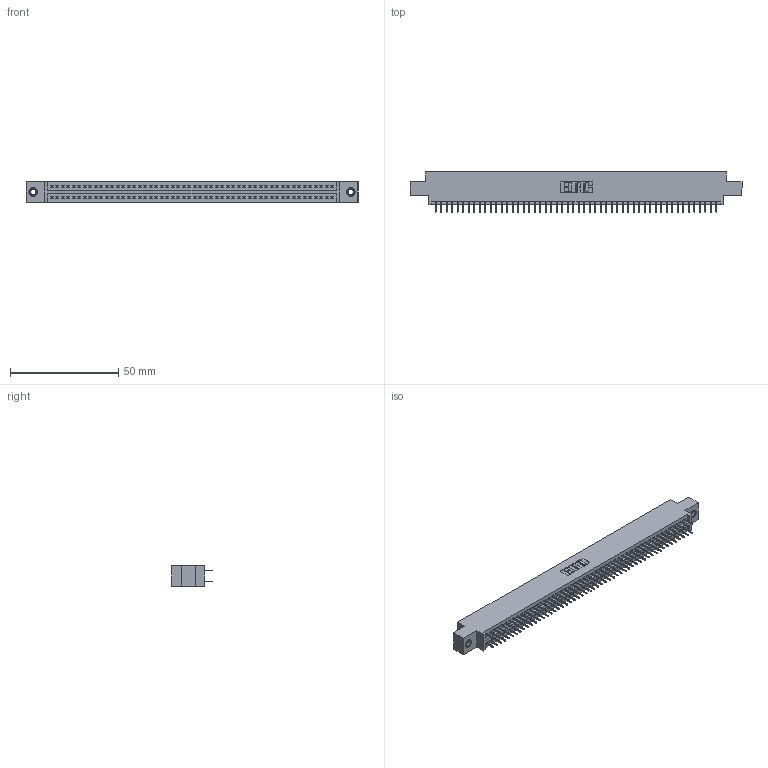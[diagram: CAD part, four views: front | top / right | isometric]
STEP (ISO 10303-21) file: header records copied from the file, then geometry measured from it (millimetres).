
FILE_DESCRIPTION (( 'STEP AP203' ), '1' );
FILE_NAME ('345-104-525-807.STEP', '2020-09-21T19:34:53', ( '' ), ( '' ), 'SwSTEP 2.0', 'SolidWorks 2020', '' );
FILE_SCHEMA (( 'CONFIG_CONTROL_DESIGN' ));
Length unit declared in the file: inch
Products named in the file (4): 345 Part_0.170 Offset - 0.156 Dia-TI; 345-250-001_345-250-005-103; 345-104-525-807; 345-292-001_345-293-125
Assembly tree (107 placements, depth 2):
  345-104-525-807
    345 Part_0.170 Offset - 0.156 Dia-TI
    345-292-001_345-293-125  x104
    345-250-001_345-250-005-103  x2
Bounding box: 153.29 x 18.72 x 9.4 mm (x, y, z)
Volume: 14685.4 mm3; surface area: 21556.7 mm2
Topology: 107 solids, 107 shells, 5806 faces, 16401 edges, 10510 vertices
Faces by surface type: plane 4172, cylinder 1618, cone 12, torus 4
Entity records: 40846 total; most frequent: CARTESIAN_POINT 6819, ORIENTED_EDGE 6746, DIRECTION 6027, EDGE_CURVE 3373, VECTOR 3017, LINE 3017, VERTEX_POINT 2240, AXIS2_PLACEMENT_3D 1505
